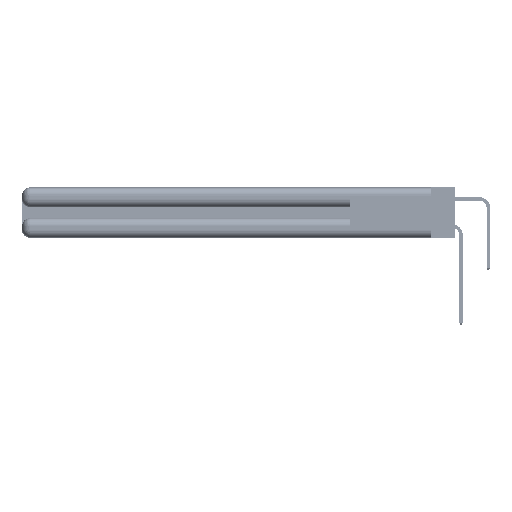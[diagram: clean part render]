
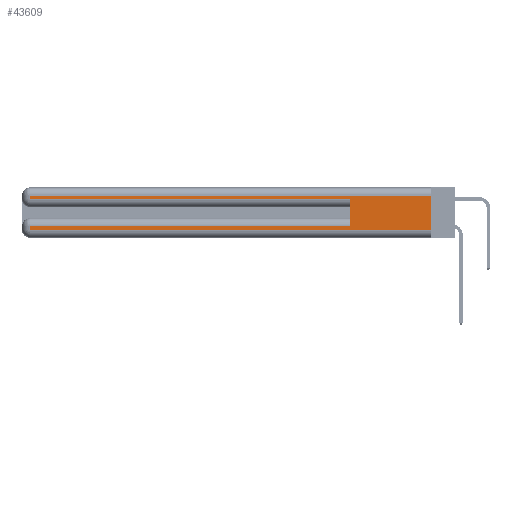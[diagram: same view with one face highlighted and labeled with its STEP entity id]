
A CAD part, left-side view. The second image highlights one B-rep face of the part: STEP entity #43609.
In plain terms, the highlighted planar face has unit normal (-1, 0, 0).
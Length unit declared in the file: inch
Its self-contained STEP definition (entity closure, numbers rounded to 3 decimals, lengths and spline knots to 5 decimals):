
#2677 = VECTOR ( 'NONE', #39321, 39.37008 ) ;
#2832 = CARTESIAN_POINT ( 'NONE',  ( 0., 0., 0.31 ) ) ;
#3932 = FACE_OUTER_BOUND ( 'NONE', #17144, .T. ) ;
#5105 = EDGE_CURVE ( 'NONE', #51810, #11939, #22606, .T. ) ;
#6451 = VECTOR ( 'NONE', #21841, 39.37008 ) ;
#7396 = CARTESIAN_POINT ( 'NONE',  ( 0., 0., 0.37 ) ) ;
#7495 = ORIENTED_EDGE ( 'NONE', *, *, #5105, .T. ) ;
#7743 = LINE ( 'NONE', #13047, #38714 ) ;
#8088 = CARTESIAN_POINT ( 'NONE',  ( 0., 2.94, 0.37 ) ) ;
#8311 = EDGE_CURVE ( 'NONE', #11939, #30199, #24257, .T. ) ;
#8444 = ORIENTED_EDGE ( 'NONE', *, *, #36378, .F. ) ;
#9167 = CARTESIAN_POINT ( 'NONE',  ( 0., 2.94, 0.31 ) ) ;
#9778 = CARTESIAN_POINT ( 'NONE',  ( 0., 0., 0.06 ) ) ;
#10103 = CARTESIAN_POINT ( 'NONE',  ( 0., 2.94, 0.06 ) ) ;
#10817 = ORIENTED_EDGE ( 'NONE', *, *, #33493, .F. ) ;
#11164 = EDGE_CURVE ( 'NONE', #37107, #32400, #40002, .T. ) ;
#11939 = VERTEX_POINT ( 'NONE', #22735 ) ;
#13047 = CARTESIAN_POINT ( 'NONE',  ( 0., 0., 0.285 ) ) ;
#13435 = LINE ( 'NONE', #8088, #33598 ) ;
#15593 = DIRECTION ( 'NONE',  ( 1., 0., 0. ) ) ;
#15906 = CARTESIAN_POINT ( 'NONE',  ( 0., 2.94, 0.37 ) ) ;
#16293 = DIRECTION ( 'NONE',  ( 0., 0., -1. ) ) ;
#16982 = LINE ( 'NONE', #50451, #35859 ) ;
#17015 = CARTESIAN_POINT ( 'NONE',  ( 0., 0.6, 0.085 ) ) ;
#17144 = EDGE_LOOP ( 'NONE', ( #8444, #38516, #37218, #40275, #10817, #7495, #18092, #33612 ) ) ;
#18092 = ORIENTED_EDGE ( 'NONE', *, *, #8311, .T. ) ;
#18639 = DIRECTION ( 'NONE',  ( 0., -1., 0. ) ) ;
#19278 = DIRECTION ( 'NONE',  ( 0., 1., 0. ) ) ;
#21841 = DIRECTION ( 'NONE',  ( 0., 1., 0. ) ) ;
#22606 = LINE ( 'NONE', #39323, #42733 ) ;
#22735 = CARTESIAN_POINT ( 'NONE',  ( 0., 2.94, 0.085 ) ) ;
#22977 = VECTOR ( 'NONE', #48103, 39.37008 ) ;
#23019 = VERTEX_POINT ( 'NONE', #38968 ) ;
#23557 = PLANE ( 'NONE',  #39922 ) ;
#24257 = LINE ( 'NONE', #15906, #22977 ) ;
#24887 = LINE ( 'NONE', #26719, #33035 ) ;
#26719 = CARTESIAN_POINT ( 'NONE',  ( 0., 0., 0.06 ) ) ;
#28086 = EDGE_CURVE ( 'NONE', #30199, #33410, #24887, .T. ) ;
#29095 = DIRECTION ( 'NONE',  ( 0., -1., 0. ) ) ;
#30199 = VERTEX_POINT ( 'NONE', #10103 ) ;
#31213 = CARTESIAN_POINT ( 'NONE',  ( 0., 0., 0.37 ) ) ;
#32400 = VERTEX_POINT ( 'NONE', #9167 ) ;
#33035 = VECTOR ( 'NONE', #18639, 39.37008 ) ;
#33410 = VERTEX_POINT ( 'NONE', #9778 ) ;
#33493 = EDGE_CURVE ( 'NONE', #51810, #23019, #16982, .T. ) ;
#33598 = VECTOR ( 'NONE', #16293, 39.37008 ) ;
#33612 = ORIENTED_EDGE ( 'NONE', *, *, #28086, .T. ) ;
#34450 = DIRECTION ( 'NONE',  ( 0., 0., 1. ) ) ;
#34940 = LINE ( 'NONE', #31213, #2677 ) ;
#35859 = VECTOR ( 'NONE', #34450, 39.37008 ) ;
#36378 = EDGE_CURVE ( 'NONE', #37107, #33410, #34940, .T. ) ;
#36734 = EDGE_CURVE ( 'NONE', #42541, #23019, #7743, .T. ) ;
#37107 = VERTEX_POINT ( 'NONE', #2832 ) ;
#37218 = ORIENTED_EDGE ( 'NONE', *, *, #37985, .T. ) ;
#37985 = EDGE_CURVE ( 'NONE', #32400, #42541, #13435, .T. ) ;
#38516 = ORIENTED_EDGE ( 'NONE', *, *, #11164, .T. ) ;
#38714 = VECTOR ( 'NONE', #29095, 39.37008 ) ;
#38968 = CARTESIAN_POINT ( 'NONE',  ( 0., 0.6, 0.285 ) ) ;
#39321 = DIRECTION ( 'NONE',  ( 0., 0., -1. ) ) ;
#39323 = CARTESIAN_POINT ( 'NONE',  ( 0., 0., 0.085 ) ) ;
#39922 = AXIS2_PLACEMENT_3D ( 'NONE', #7396, #15593, #43781 ) ;
#40002 = LINE ( 'NONE', #45909, #6451 ) ;
#40275 = ORIENTED_EDGE ( 'NONE', *, *, #36734, .T. ) ;
#42541 = VERTEX_POINT ( 'NONE', #48793 ) ;
#42733 = VECTOR ( 'NONE', #19278, 39.37008 ) ;
#43609 = ADVANCED_FACE ( 'NONE', ( #3932 ), #23557, .F. ) ;
#43781 = DIRECTION ( 'NONE',  ( 0., 0., -1. ) ) ;
#45909 = CARTESIAN_POINT ( 'NONE',  ( 0., 0., 0.31 ) ) ;
#48103 = DIRECTION ( 'NONE',  ( 0., 0., -1. ) ) ;
#48793 = CARTESIAN_POINT ( 'NONE',  ( 0., 2.94, 0.285 ) ) ;
#50451 = CARTESIAN_POINT ( 'NONE',  ( 0., 0.6, 0.145 ) ) ;
#51810 = VERTEX_POINT ( 'NONE', #17015 ) ;
